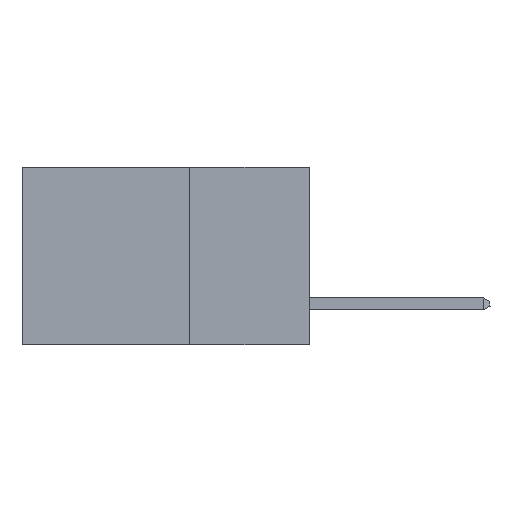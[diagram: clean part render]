
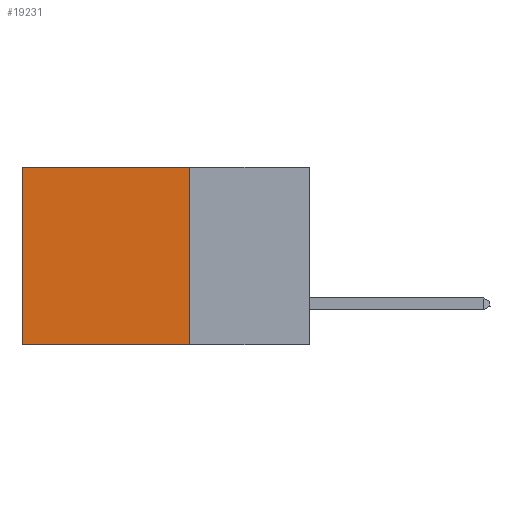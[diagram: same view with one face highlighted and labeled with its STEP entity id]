
A CAD part, left-side view. The second image highlights one B-rep face of the part: STEP entity #19231.
In plain terms, the highlighted planar face has unit normal (-1, 0, 0).
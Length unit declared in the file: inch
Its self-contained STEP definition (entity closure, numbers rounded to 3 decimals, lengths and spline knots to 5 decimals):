
#215 = FACE_OUTER_BOUND ( 'NONE', #20495, .T. ) ;
#273 = CARTESIAN_POINT ( 'NONE',  ( 0.2875, 0.6, -0.37 ) ) ;
#347 = CARTESIAN_POINT ( 'NONE',  ( 0.2875, 0.25, 0. ) ) ;
#1068 = CARTESIAN_POINT ( 'NONE',  ( 0.2875, 0.25, 0. ) ) ;
#2017 = CARTESIAN_POINT ( 'NONE',  ( 0.2875, 0.6, 0. ) ) ;
#2462 = CARTESIAN_POINT ( 'NONE',  ( 0.2875, 0.25, -0.37 ) ) ;
#3123 = DIRECTION ( 'NONE',  ( 1., 0., 0. ) ) ;
#3953 = DIRECTION ( 'NONE',  ( 0., 0., -1. ) ) ;
#3965 = ORIENTED_EDGE ( 'NONE', *, *, #11401, .T. ) ;
#4852 = VECTOR ( 'NONE', #3953, 39.37008 ) ;
#6390 = EDGE_CURVE ( 'NONE', #19706, #12763, #9925, .T. ) ;
#8077 = ORIENTED_EDGE ( 'NONE', *, *, #10935, .F. ) ;
#8806 = CARTESIAN_POINT ( 'NONE',  ( 0.2875, 0.6, 0. ) ) ;
#9925 = LINE ( 'NONE', #347, #4852 ) ;
#10935 = EDGE_CURVE ( 'NONE', #12763, #16647, #16617, .T. ) ;
#11401 = EDGE_CURVE ( 'NONE', #13741, #16647, #19552, .T. ) ;
#11879 = CARTESIAN_POINT ( 'NONE',  ( 0.2875, 0.25, -0.37 ) ) ;
#12607 = DIRECTION ( 'NONE',  ( 0., 0., -1. ) ) ;
#12763 = VERTEX_POINT ( 'NONE', #11879 ) ;
#12807 = EDGE_CURVE ( 'NONE', #19706, #13741, #22237, .T. ) ;
#13741 = VERTEX_POINT ( 'NONE', #2017 ) ;
#13953 = DIRECTION ( 'NONE',  ( 0., 1., 0. ) ) ;
#14568 = CARTESIAN_POINT ( 'NONE',  ( 0.2875, 0.25, 0. ) ) ;
#15061 = VECTOR ( 'NONE', #12607, 39.37008 ) ;
#15352 = DIRECTION ( 'NONE',  ( 0., 1., 0. ) ) ;
#16524 = VECTOR ( 'NONE', #15352, 39.37008 ) ;
#16617 = LINE ( 'NONE', #2462, #23884 ) ;
#16647 = VERTEX_POINT ( 'NONE', #273 ) ;
#17337 = CARTESIAN_POINT ( 'NONE',  ( 0.2875, 0.25, 0. ) ) ;
#17933 = ORIENTED_EDGE ( 'NONE', *, *, #6390, .F. ) ;
#18489 = AXIS2_PLACEMENT_3D ( 'NONE', #14568, #3123, #22361 ) ;
#18491 = PLANE ( 'NONE',  #18489 ) ;
#19231 = ADVANCED_FACE ( 'NONE', ( #215 ), #18491, .F. ) ;
#19552 = LINE ( 'NONE', #8806, #15061 ) ;
#19706 = VERTEX_POINT ( 'NONE', #1068 ) ;
#20495 = EDGE_LOOP ( 'NONE', ( #3965, #8077, #17933, #24278 ) ) ;
#22237 = LINE ( 'NONE', #17337, #16524 ) ;
#22361 = DIRECTION ( 'NONE',  ( 0., 0., -1. ) ) ;
#23884 = VECTOR ( 'NONE', #13953, 39.37008 ) ;
#24278 = ORIENTED_EDGE ( 'NONE', *, *, #12807, .T. ) ;
